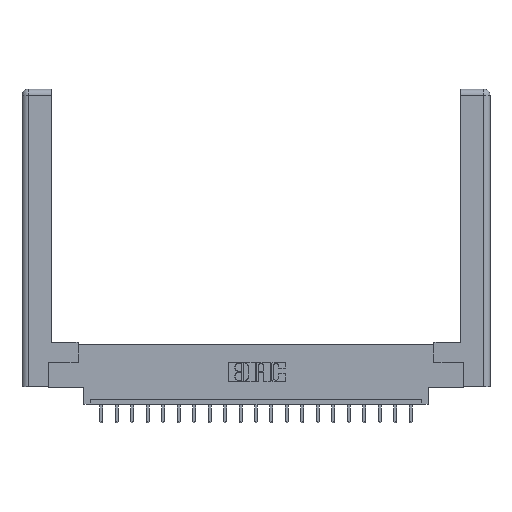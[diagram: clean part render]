
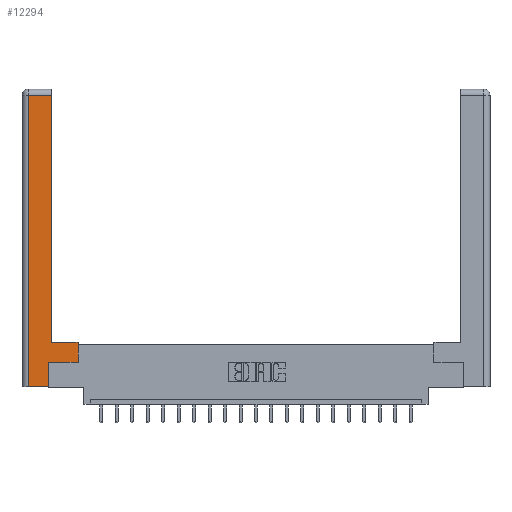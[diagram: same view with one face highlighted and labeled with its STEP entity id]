
A CAD part, top view. The second image highlights one B-rep face of the part: STEP entity #12294.
In plain terms, the highlighted planar face has unit normal (0, 0, 1).
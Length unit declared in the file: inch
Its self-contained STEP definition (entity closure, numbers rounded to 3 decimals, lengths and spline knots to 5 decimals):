
#15 = ORIENTED_EDGE ( 'NONE', *, *, #17513, .T. ) ;
#105 = ORIENTED_EDGE ( 'NONE', *, *, #16384, .T. ) ;
#273 = VERTEX_POINT ( 'NONE', #16976 ) ;
#311 = CARTESIAN_POINT ( 'NONE',  ( 0.295, 2.94, 0. ) ) ;
#315 = CARTESIAN_POINT ( 'NONE',  ( 0.0615, 0., 0. ) ) ;
#381 = CARTESIAN_POINT ( 'NONE',  ( 0.265, 0.245, 0. ) ) ;
#841 = CARTESIAN_POINT ( 'NONE',  ( 0.295, 0.45, 0. ) ) ;
#1438 = AXIS2_PLACEMENT_3D ( 'NONE', #1946, #13397, #6804 ) ;
#1635 = DIRECTION ( 'NONE',  ( 0., 1., 0. ) ) ;
#1799 = LINE ( 'NONE', #19666, #9491 ) ;
#1946 = CARTESIAN_POINT ( 'NONE',  ( 0., 0., 0. ) ) ;
#2117 = VERTEX_POINT ( 'NONE', #5677 ) ;
#2689 = LINE ( 'NONE', #9480, #12437 ) ;
#2906 = EDGE_CURVE ( 'NONE', #4632, #10332, #14088, .T. ) ;
#3116 = EDGE_CURVE ( 'NONE', #19724, #4632, #1799, .T. ) ;
#3521 = ORIENTED_EDGE ( 'NONE', *, *, #21041, .T. ) ;
#3673 = CARTESIAN_POINT ( 'NONE',  ( 0.0615, 0., 0. ) ) ;
#4050 = CARTESIAN_POINT ( 'NONE',  ( 0.265, 0., 0. ) ) ;
#4116 = DIRECTION ( 'NONE',  ( -1., 0., 0. ) ) ;
#4621 = VERTEX_POINT ( 'NONE', #381 ) ;
#4632 = VERTEX_POINT ( 'NONE', #311 ) ;
#5119 = CARTESIAN_POINT ( 'NONE',  ( 0.565, 0.45, 0. ) ) ;
#5139 = PLANE ( 'NONE',  #1438 ) ;
#5357 = ORIENTED_EDGE ( 'NONE', *, *, #14174, .T. ) ;
#5553 = LINE ( 'NONE', #5119, #16596 ) ;
#5677 = CARTESIAN_POINT ( 'NONE',  ( 0.565, 0.245, 0. ) ) ;
#5927 = CARTESIAN_POINT ( 'NONE',  ( 0.0615, 2.94, 0. ) ) ;
#6461 = EDGE_LOOP ( 'NONE', ( #15486, #20440, #5357, #3521, #15, #18333, #10984, #105 ) ) ;
#6804 = DIRECTION ( 'NONE',  ( -1., 0., 0. ) ) ;
#7225 = VECTOR ( 'NONE', #7601, 39.37008 ) ;
#7601 = DIRECTION ( 'NONE',  ( 0., 1., 0. ) ) ;
#7814 = VECTOR ( 'NONE', #4116, 39.37008 ) ;
#9036 = DIRECTION ( 'NONE',  ( 1., 0., 0. ) ) ;
#9422 = EDGE_CURVE ( 'NONE', #2117, #16831, #5553, .T. ) ;
#9480 = CARTESIAN_POINT ( 'NONE',  ( 0.565, 0.245, 0. ) ) ;
#9491 = VECTOR ( 'NONE', #1635, 39.37008 ) ;
#9763 = VECTOR ( 'NONE', #18898, 39.37008 ) ;
#9793 = CARTESIAN_POINT ( 'NONE',  ( 0.0615, 2.94, 0. ) ) ;
#9947 = LINE ( 'NONE', #3673, #18140 ) ;
#10332 = VERTEX_POINT ( 'NONE', #9793 ) ;
#10645 = LINE ( 'NONE', #4050, #21095 ) ;
#10984 = ORIENTED_EDGE ( 'NONE', *, *, #9422, .T. ) ;
#10986 = CARTESIAN_POINT ( 'NONE',  ( 0.265, 0.245, 0. ) ) ;
#11734 = DIRECTION ( 'NONE',  ( 0., 1., 0. ) ) ;
#12294 = ADVANCED_FACE ( 'NONE', ( #15946 ), #5139, .F. ) ;
#12437 = VECTOR ( 'NONE', #14484, 39.37008 ) ;
#13397 = DIRECTION ( 'NONE',  ( 0., 0., -1. ) ) ;
#13613 = CARTESIAN_POINT ( 'NONE',  ( 0.295, 0.45, 0. ) ) ;
#14088 = LINE ( 'NONE', #5927, #9763 ) ;
#14174 = EDGE_CURVE ( 'NONE', #10332, #17123, #9947, .T. ) ;
#14484 = DIRECTION ( 'NONE',  ( 1., 0., 0. ) ) ;
#15486 = ORIENTED_EDGE ( 'NONE', *, *, #3116, .T. ) ;
#15946 = FACE_OUTER_BOUND ( 'NONE', #6461, .T. ) ;
#16384 = EDGE_CURVE ( 'NONE', #16831, #19724, #20087, .T. ) ;
#16596 = VECTOR ( 'NONE', #11734, 39.37008 ) ;
#16721 = CARTESIAN_POINT ( 'NONE',  ( 0.565, 0.45, 0. ) ) ;
#16831 = VERTEX_POINT ( 'NONE', #16721 ) ;
#16976 = CARTESIAN_POINT ( 'NONE',  ( 0.265, 0., 0. ) ) ;
#17123 = VERTEX_POINT ( 'NONE', #315 ) ;
#17513 = EDGE_CURVE ( 'NONE', #273, #4621, #21046, .T. ) ;
#18140 = VECTOR ( 'NONE', #18447, 39.37008 ) ;
#18333 = ORIENTED_EDGE ( 'NONE', *, *, #20715, .T. ) ;
#18447 = DIRECTION ( 'NONE',  ( 0., -1., 0. ) ) ;
#18898 = DIRECTION ( 'NONE',  ( -1., 0., 0. ) ) ;
#19666 = CARTESIAN_POINT ( 'NONE',  ( 0.295, 3., 0. ) ) ;
#19724 = VERTEX_POINT ( 'NONE', #13613 ) ;
#20087 = LINE ( 'NONE', #841, #7814 ) ;
#20440 = ORIENTED_EDGE ( 'NONE', *, *, #2906, .T. ) ;
#20715 = EDGE_CURVE ( 'NONE', #4621, #2117, #2689, .T. ) ;
#21041 = EDGE_CURVE ( 'NONE', #17123, #273, #10645, .T. ) ;
#21046 = LINE ( 'NONE', #10986, #7225 ) ;
#21095 = VECTOR ( 'NONE', #9036, 39.37008 ) ;
